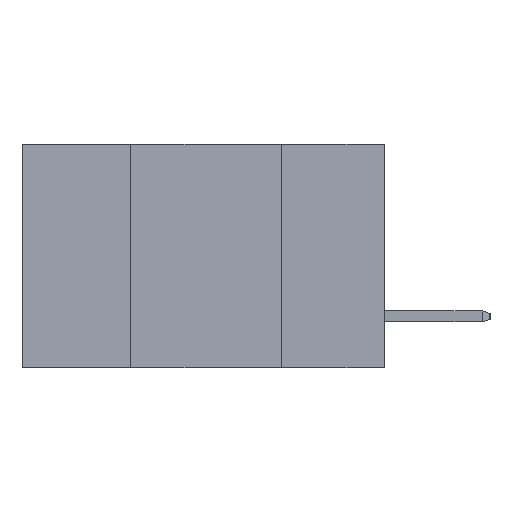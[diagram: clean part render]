
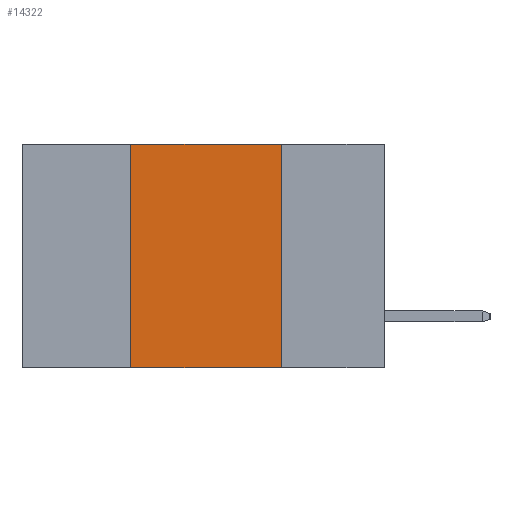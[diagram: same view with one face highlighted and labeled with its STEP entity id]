
A CAD part, left-side view. The second image highlights one B-rep face of the part: STEP entity #14322.
In plain terms, the highlighted planar face has unit normal (-1, 0, 0).
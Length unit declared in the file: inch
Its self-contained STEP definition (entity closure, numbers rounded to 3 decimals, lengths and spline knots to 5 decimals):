
#937 = ORIENTED_EDGE ( 'NONE', *, *, #17350, .F. ) ;
#1646 = DIRECTION ( 'NONE',  ( 0., 0., -1. ) ) ;
#2088 = VERTEX_POINT ( 'NONE', #6222 ) ;
#2992 = DIRECTION ( 'NONE',  ( 0., 0., 1. ) ) ;
#5013 = VECTOR ( 'NONE', #1646, 39.37008 ) ;
#5071 = DIRECTION ( 'NONE',  ( 0., -1., 0. ) ) ;
#5085 = DIRECTION ( 'NONE',  ( 0., 0., -1. ) ) ;
#5126 = VECTOR ( 'NONE', #2992, 39.37008 ) ;
#5681 = LINE ( 'NONE', #13493, #5126 ) ;
#5819 = VECTOR ( 'NONE', #5071, 39.37008 ) ;
#6222 = CARTESIAN_POINT ( 'NONE',  ( 0., 0.17, 0. ) ) ;
#6671 = CARTESIAN_POINT ( 'NONE',  ( 0., 0.42, 0. ) ) ;
#8482 = CARTESIAN_POINT ( 'NONE',  ( 0., 0.6, -0.37 ) ) ;
#10183 = VERTEX_POINT ( 'NONE', #18175 ) ;
#10547 = LINE ( 'NONE', #15398, #5819 ) ;
#10939 = EDGE_LOOP ( 'NONE', ( #12849, #22023, #937, #15432 ) ) ;
#11089 = FACE_OUTER_BOUND ( 'NONE', #10939, .T. ) ;
#11831 = LINE ( 'NONE', #8482, #15691 ) ;
#12090 = CARTESIAN_POINT ( 'NONE',  ( 0., 0.6, 0. ) ) ;
#12849 = ORIENTED_EDGE ( 'NONE', *, *, #13786, .F. ) ;
#13493 = CARTESIAN_POINT ( 'NONE',  ( 0., 0.42, 0. ) ) ;
#13690 = PLANE ( 'NONE',  #15946 ) ;
#13786 = EDGE_CURVE ( 'NONE', #2088, #10183, #14233, .T. ) ;
#14233 = LINE ( 'NONE', #22034, #5013 ) ;
#14322 = ADVANCED_FACE ( 'NONE', ( #11089 ), #13690, .F. ) ;
#14889 = EDGE_CURVE ( 'NONE', #18820, #2088, #10547, .T. ) ;
#15398 = CARTESIAN_POINT ( 'NONE',  ( 0., 0.6, 0. ) ) ;
#15418 = DIRECTION ( 'NONE',  ( 1., 0., 0. ) ) ;
#15432 = ORIENTED_EDGE ( 'NONE', *, *, #18861, .T. ) ;
#15691 = VECTOR ( 'NONE', #16925, 39.37008 ) ;
#15946 = AXIS2_PLACEMENT_3D ( 'NONE', #12090, #15418, #5085 ) ;
#16925 = DIRECTION ( 'NONE',  ( 0., -1., 0. ) ) ;
#17350 = EDGE_CURVE ( 'NONE', #22045, #18820, #5681, .T. ) ;
#18175 = CARTESIAN_POINT ( 'NONE',  ( 0., 0.17, -0.37 ) ) ;
#18820 = VERTEX_POINT ( 'NONE', #6671 ) ;
#18861 = EDGE_CURVE ( 'NONE', #22045, #10183, #11831, .T. ) ;
#21951 = CARTESIAN_POINT ( 'NONE',  ( 0., 0.42, -0.37 ) ) ;
#22023 = ORIENTED_EDGE ( 'NONE', *, *, #14889, .F. ) ;
#22034 = CARTESIAN_POINT ( 'NONE',  ( 0., 0.17, 0. ) ) ;
#22045 = VERTEX_POINT ( 'NONE', #21951 ) ;
